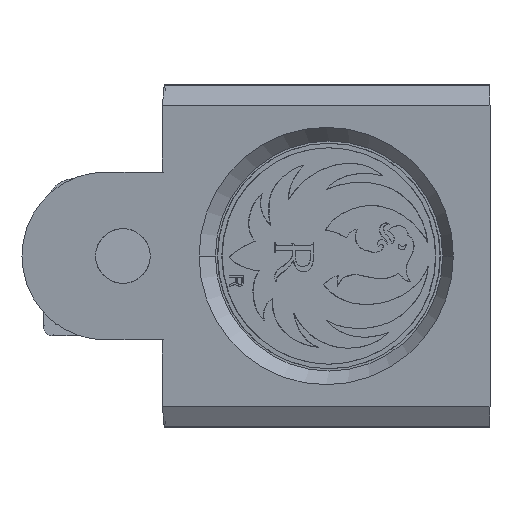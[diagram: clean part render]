
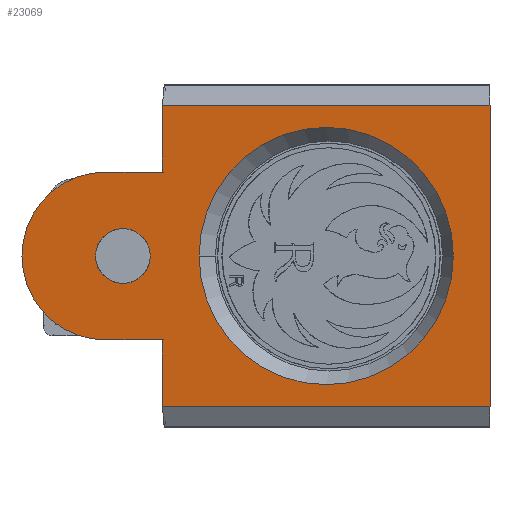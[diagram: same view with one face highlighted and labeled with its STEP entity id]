
A CAD part, front view. The second image highlights one B-rep face of the part: STEP entity #23069.
In plain terms, the highlighted face is planar.
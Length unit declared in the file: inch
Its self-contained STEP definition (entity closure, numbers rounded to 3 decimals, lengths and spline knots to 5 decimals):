
#19075=DIRECTION('',(-1.,0.,0.));
#19076=VECTOR('',#19075,0.728);
#19077=CARTESIAN_POINT('',(0.364,0.,-0.33071));
#19078=LINE('',#19077,#19076);
#19082=DIRECTION('',(0.,0.,1.));
#19083=VECTOR('',#19082,0.14671);
#19084=CARTESIAN_POINT('',(-0.364,0.,-0.33071));
#19085=LINE('',#19084,#19083);
#19089=DIRECTION('',(-1.,0.,0.));
#19090=VECTOR('',#19089,0.128);
#19091=CARTESIAN_POINT('',(-0.364,0.,-0.184));
#19092=LINE('',#19091,#19090);
#19096=CARTESIAN_POINT('',(-0.492,0.,0.));
#19097=DIRECTION('',(0.,1.,0.));
#19098=DIRECTION('',(0.,0.,-1.));
#19099=AXIS2_PLACEMENT_3D('',#19096,#19097,#19098);
#19104=DIRECTION('',(1.,0.,0.));
#19105=VECTOR('',#19104,0.128);
#19106=CARTESIAN_POINT('',(-0.492,0.,0.184));
#19107=LINE('',#19106,#19105);
#19111=DIRECTION('',(0.,0.,1.));
#19112=VECTOR('',#19111,0.14671);
#19113=CARTESIAN_POINT('',(-0.364,0.,0.184));
#19114=LINE('',#19113,#19112);
#19118=DIRECTION('',(-1.,0.,0.));
#19119=VECTOR('',#19118,0.728);
#19120=CARTESIAN_POINT('',(0.364,0.,0.33071));
#19121=LINE('',#19120,#19119);
#19125=CARTESIAN_POINT('',(-0.391,0.,0.));
#19126=CARTESIAN_POINT('',(-0.391,0.,0.00707));
#19127=CARTESIAN_POINT('',(-0.39359,0.,0.02235));
#19128=CARTESIAN_POINT('',(-0.40752,0.,0.0437));
#19129=CARTESIAN_POINT('',(-0.42549,0.,0.05514));
#19130=CARTESIAN_POINT('',(-0.44078,0.,0.05937));
#19131=CARTESIAN_POINT('',(-0.45175,0.,0.06032));
#19132=CARTESIAN_POINT('',(-0.46272,0.,0.05937));
#19133=CARTESIAN_POINT('',(-0.47801,0.,0.05514));
#19134=CARTESIAN_POINT('',(-0.49598,0.,0.0437));
#19135=CARTESIAN_POINT('',(-0.5099,0.,0.02235));
#19136=CARTESIAN_POINT('',(-0.5125,0.,0.00707));
#19137=CARTESIAN_POINT('',(-0.5125,0.,0.));
#19142=CARTESIAN_POINT('',(-0.5125,0.,0.));
#19143=CARTESIAN_POINT('',(-0.5125,0.,-0.00707));
#19144=CARTESIAN_POINT('',(-0.5099,0.,-0.02235));
#19145=CARTESIAN_POINT('',(-0.49598,0.,-0.0437));
#19146=CARTESIAN_POINT('',(-0.47801,0.,-0.05514));
#19147=CARTESIAN_POINT('',(-0.46272,0.,-0.05937));
#19148=CARTESIAN_POINT('',(-0.45175,0.,-0.06032));
#19149=CARTESIAN_POINT('',(-0.44078,0.,-0.05937));
#19150=CARTESIAN_POINT('',(-0.42549,0.,-0.05514));
#19151=CARTESIAN_POINT('',(-0.40752,0.,-0.0437));
#19152=CARTESIAN_POINT('',(-0.39359,0.,-0.02235));
#19153=CARTESIAN_POINT('',(-0.391,0.,-0.00707));
#19154=CARTESIAN_POINT('',(-0.391,0.,0.));
#19159=CARTESIAN_POINT('',(0.,0.,0.));
#19160=DIRECTION('',(0.,-1.,0.));
#19161=DIRECTION('',(1.,0.,0.));
#19162=AXIS2_PLACEMENT_3D('',#19159,#19160,#19161);
#19167=CARTESIAN_POINT('',(0.,0.,0.));
#19168=DIRECTION('',(0.,-1.,0.));
#19169=DIRECTION('',(-1.,0.,0.));
#19170=AXIS2_PLACEMENT_3D('',#19167,#19168,#19169);
#19182=DIRECTION('',(0.,0.,1.));
#19183=VECTOR('',#19182,0.66141);
#19184=CARTESIAN_POINT('',(0.364,0.,-0.33071));
#19185=LINE('',#19184,#19183);
#22567=CARTESIAN_POINT('',(-0.364,0.,-0.184));
#22568=CARTESIAN_POINT('',(-0.492,0.,-0.184));
#22569=VERTEX_POINT('',#22567);
#22570=VERTEX_POINT('',#22568);
#22571=CARTESIAN_POINT('',(-0.492,0.,0.184));
#22572=VERTEX_POINT('',#22571);
#22573=CARTESIAN_POINT('',(-0.364,0.,0.184));
#22574=VERTEX_POINT('',#22573);
#22623=CARTESIAN_POINT('',(0.364,0.,-0.33071));
#22624=CARTESIAN_POINT('',(-0.364,0.,-0.33071));
#22625=VERTEX_POINT('',#22623);
#22626=VERTEX_POINT('',#22624);
#22671=CARTESIAN_POINT('',(-0.364,0.,0.33071));
#22672=VERTEX_POINT('',#22671);
#22679=CARTESIAN_POINT('',(0.364,0.,0.33071));
#22680=VERTEX_POINT('',#22679);
#22731=VERTEX_POINT('',#19125);
#22732=VERTEX_POINT('',#19137);
#22739=CARTESIAN_POINT('',(0.2825,0.,0.));
#22740=CARTESIAN_POINT('',(-0.2825,0.,0.));
#22741=VERTEX_POINT('',#22739);
#22742=VERTEX_POINT('',#22740);
#23034=CARTESIAN_POINT('',(0.,0.,0.));
#23035=DIRECTION('',(0.,1.,0.));
#23036=DIRECTION('',(1.,0.,0.));
#23037=AXIS2_PLACEMENT_3D('',#23034,#23035,#23036);
#23038=PLANE('',#23037);
#23040=ORIENTED_EDGE('',*,*,#23039,.T.);
#23042=ORIENTED_EDGE('',*,*,#23041,.T.);
#23044=ORIENTED_EDGE('',*,*,#23043,.T.);
#23046=ORIENTED_EDGE('',*,*,#23045,.T.);
#23048=ORIENTED_EDGE('',*,*,#23047,.T.);
#23050=ORIENTED_EDGE('',*,*,#23049,.T.);
#23052=ORIENTED_EDGE('',*,*,#23051,.F.);
#23054=ORIENTED_EDGE('',*,*,#23053,.F.);
#23055=EDGE_LOOP('',(#23040,#23042,#23044,#23046,#23048,#23050,#23052,#23054));
#23056=FACE_OUTER_BOUND('',#23055,.F.);
#23058=ORIENTED_EDGE('',*,*,#23057,.T.);
#23060=ORIENTED_EDGE('',*,*,#23059,.T.);
#23061=EDGE_LOOP('',(#23058,#23060));
#23062=FACE_BOUND('',#23061,.F.);
#23064=ORIENTED_EDGE('',*,*,#23063,.T.);
#23066=ORIENTED_EDGE('',*,*,#23065,.T.);
#23067=EDGE_LOOP('',(#23064,#23066));
#23068=FACE_BOUND('',#23067,.F.);
#23069=ADVANCED_FACE('',(#23056,#23062,#23068),#23038,.F.);
#19100=CIRCLE('',#19099,0.184);
#19138=B_SPLINE_CURVE_WITH_KNOTS('',3,(#19125,#19126,#19127,#19128,#19129,
#19130,#19131,#19132,#19133,#19134,#19135,#19136,#19137),.UNSPECIFIED.,.F.,.F.,(
4,1,1,1,1,1,1,1,1,1,4),(0.,0.125,0.25,0.375,0.4375,0.5,0.5625,
0.625,0.75,0.875,1.),.UNSPECIFIED.);
#19155=B_SPLINE_CURVE_WITH_KNOTS('',3,(#19142,#19143,#19144,#19145,#19146,
#19147,#19148,#19149,#19150,#19151,#19152,#19153,#19154),.UNSPECIFIED.,.F.,.F.,(
4,1,1,1,1,1,1,1,1,1,4),(0.,0.125,0.25,0.375,0.4375,0.5,0.5625,
0.625,0.75,0.875,1.),.UNSPECIFIED.);
#19163=CIRCLE('',#19162,0.2825);
#19171=CIRCLE('',#19170,0.2825);
#23039=EDGE_CURVE('',#22625,#22626,#19078,.T.);
#23041=EDGE_CURVE('',#22626,#22569,#19085,.T.);
#23043=EDGE_CURVE('',#22569,#22570,#19092,.T.);
#23045=EDGE_CURVE('',#22570,#22572,#19100,.T.);
#23047=EDGE_CURVE('',#22572,#22574,#19107,.T.);
#23049=EDGE_CURVE('',#22574,#22672,#19114,.T.);
#23051=EDGE_CURVE('',#22680,#22672,#19121,.T.);
#23053=EDGE_CURVE('',#22625,#22680,#19185,.T.);
#23057=EDGE_CURVE('',#22731,#22732,#19138,.T.);
#23059=EDGE_CURVE('',#22732,#22731,#19155,.T.);
#23063=EDGE_CURVE('',#22741,#22742,#19163,.T.);
#23065=EDGE_CURVE('',#22742,#22741,#19171,.T.);
